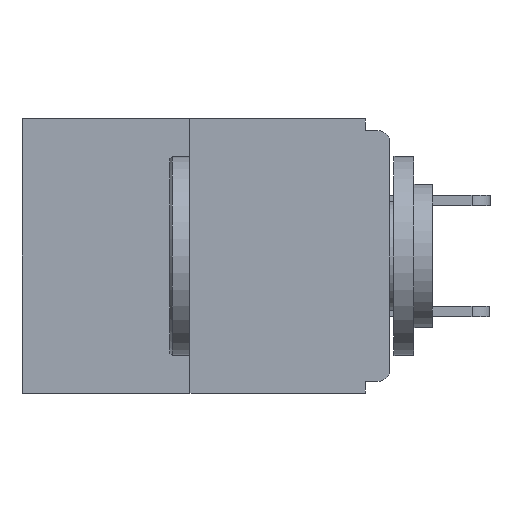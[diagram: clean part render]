
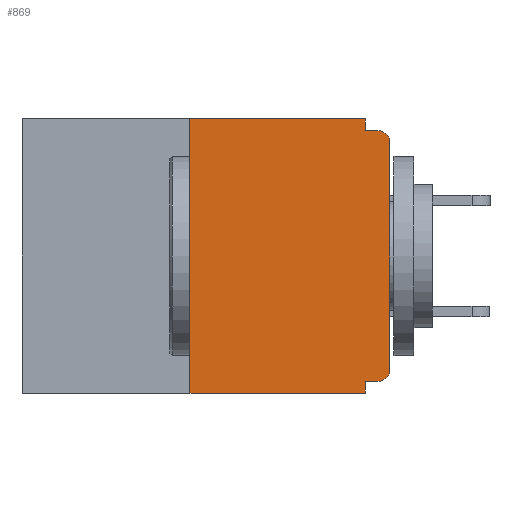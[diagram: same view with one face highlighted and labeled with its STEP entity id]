
A CAD part, left-side view. The second image highlights one B-rep face of the part: STEP entity #869.
In plain terms, the highlighted planar face has unit normal (-1, 0, 0).
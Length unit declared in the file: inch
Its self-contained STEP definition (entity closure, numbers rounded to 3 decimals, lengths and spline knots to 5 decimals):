
#82 = DIRECTION ( 'NONE',  ( 0., -1., 0. ) ) ;
#92 = ORIENTED_EDGE ( 'NONE', *, *, #14170, .T. ) ;
#514 = DIRECTION ( 'NONE',  ( 0., 0., -1. ) ) ;
#869 = ADVANCED_FACE ( 'NONE', ( #8161 ), #7181, .F. ) ;
#1082 = VECTOR ( 'NONE', #12350, 39.37008 ) ;
#1517 = VECTOR ( 'NONE', #14670, 39.37008 ) ;
#1728 = AXIS2_PLACEMENT_3D ( 'NONE', #14486, #8746, #17326 ) ;
#1764 = DIRECTION ( 'NONE',  ( -1., 0., 0. ) ) ;
#2073 = CARTESIAN_POINT ( 'NONE',  ( 0., 0.031, 0. ) ) ;
#2303 = LINE ( 'NONE', #11290, #13924 ) ;
#2343 = CARTESIAN_POINT ( 'NONE',  ( 0., 0.46, -0.343 ) ) ;
#2442 = EDGE_CURVE ( 'NONE', #13211, #17263, #9874, .T. ) ;
#2461 = AXIS2_PLACEMENT_3D ( 'NONE', #17201, #5905, #3043 ) ;
#2674 = VECTOR ( 'NONE', #3726, 39.37008 ) ;
#2774 = ORIENTED_EDGE ( 'NONE', *, *, #2442, .T. ) ;
#3043 = DIRECTION ( 'NONE',  ( 0., 0., -1. ) ) ;
#3223 = VECTOR ( 'NONE', #10202, 39.37008 ) ;
#3483 = CARTESIAN_POINT ( 'NONE',  ( 0., 0.031, -0.343 ) ) ;
#3511 = CARTESIAN_POINT ( 'NONE',  ( 0., 0.46, 0. ) ) ;
#3658 = CARTESIAN_POINT ( 'NONE',  ( 0., 0.25, 0. ) ) ;
#3726 = DIRECTION ( 'NONE',  ( 0., 0., 1. ) ) ;
#4218 = LINE ( 'NONE', #3658, #2674 ) ;
#4371 = CARTESIAN_POINT ( 'NONE',  ( 0., 0.25, -0.343 ) ) ;
#4703 = CARTESIAN_POINT ( 'NONE',  ( 0., 0., -0.328 ) ) ;
#4836 = EDGE_CURVE ( 'NONE', #18146, #11204, #14494, .T. ) ;
#5706 = CARTESIAN_POINT ( 'NONE',  ( 0., 0.031, -0.328 ) ) ;
#5816 = VERTEX_POINT ( 'NONE', #4371 ) ;
#5905 = DIRECTION ( 'NONE',  ( -1., 0., 0. ) ) ;
#5981 = CARTESIAN_POINT ( 'NONE',  ( 0., 0., -0.313 ) ) ;
#6450 = VECTOR ( 'NONE', #12423, 39.37008 ) ;
#7181 = PLANE ( 'NONE',  #1728 ) ;
#7378 = VECTOR ( 'NONE', #15451, 39.37008 ) ;
#7770 = DIRECTION ( 'NONE',  ( 0., -1., 0. ) ) ;
#7812 = LINE ( 'NONE', #4703, #1517 ) ;
#8161 = FACE_OUTER_BOUND ( 'NONE', #9070, .T. ) ;
#8279 = CARTESIAN_POINT ( 'NONE',  ( 0., 0.031, 0. ) ) ;
#8521 = EDGE_CURVE ( 'NONE', #18119, #12686, #9248, .T. ) ;
#8746 = DIRECTION ( 'NONE',  ( 1., 0., 0. ) ) ;
#8835 = CARTESIAN_POINT ( 'NONE',  ( 0., 0., 0. ) ) ;
#8848 = EDGE_CURVE ( 'NONE', #9846, #17263, #2303, .T. ) ;
#9070 = EDGE_LOOP ( 'NONE', ( #9831, #10696, #92, #11551, #13028, #14456, #15803, #2774, #17605, #9783 ) ) ;
#9082 = CARTESIAN_POINT ( 'NONE',  ( 0., 0.031, -0.015 ) ) ;
#9248 = LINE ( 'NONE', #3511, #14383 ) ;
#9339 = CARTESIAN_POINT ( 'NONE',  ( 0., 0.015, -0.328 ) ) ;
#9377 = LINE ( 'NONE', #2343, #1082 ) ;
#9783 = ORIENTED_EDGE ( 'NONE', *, *, #13656, .F. ) ;
#9831 = ORIENTED_EDGE ( 'NONE', *, *, #8521, .F. ) ;
#9846 = VERTEX_POINT ( 'NONE', #9082 ) ;
#9874 = CIRCLE ( 'NONE', #17698, 0.015 ) ;
#10202 = DIRECTION ( 'NONE',  ( 0., 0., 1. ) ) ;
#10339 = CARTESIAN_POINT ( 'NONE',  ( 0., 0.015, -0.03 ) ) ;
#10652 = EDGE_CURVE ( 'NONE', #11870, #18146, #7812, .T. ) ;
#10696 = ORIENTED_EDGE ( 'NONE', *, *, #13470, .F. ) ;
#10851 = CARTESIAN_POINT ( 'NONE',  ( 0., 0.031, -0.343 ) ) ;
#10976 = EDGE_CURVE ( 'NONE', #11870, #16475, #16549, .T. ) ;
#11204 = VERTEX_POINT ( 'NONE', #3483 ) ;
#11290 = CARTESIAN_POINT ( 'NONE',  ( 0., 0., -0.015 ) ) ;
#11551 = ORIENTED_EDGE ( 'NONE', *, *, #4836, .F. ) ;
#11870 = VERTEX_POINT ( 'NONE', #9339 ) ;
#12014 = CARTESIAN_POINT ( 'NONE',  ( 0., 0., -0.03 ) ) ;
#12350 = DIRECTION ( 'NONE',  ( 0., -1., 0. ) ) ;
#12423 = DIRECTION ( 'NONE',  ( 0., 0., -1. ) ) ;
#12686 = VERTEX_POINT ( 'NONE', #2073 ) ;
#13028 = ORIENTED_EDGE ( 'NONE', *, *, #10652, .F. ) ;
#13211 = VERTEX_POINT ( 'NONE', #12014 ) ;
#13292 = LINE ( 'NONE', #8835, #3223 ) ;
#13470 = EDGE_CURVE ( 'NONE', #5816, #18119, #4218, .T. ) ;
#13656 = EDGE_CURVE ( 'NONE', #12686, #9846, #15001, .T. ) ;
#13924 = VECTOR ( 'NONE', #82, 39.37008 ) ;
#14088 = CARTESIAN_POINT ( 'NONE',  ( 0., 0.25, 0. ) ) ;
#14170 = EDGE_CURVE ( 'NONE', #5816, #11204, #9377, .T. ) ;
#14383 = VECTOR ( 'NONE', #7770, 39.37008 ) ;
#14456 = ORIENTED_EDGE ( 'NONE', *, *, #10976, .T. ) ;
#14486 = CARTESIAN_POINT ( 'NONE',  ( 0., 0.46, 0. ) ) ;
#14494 = LINE ( 'NONE', #10851, #6450 ) ;
#14670 = DIRECTION ( 'NONE',  ( 0., 1., 0. ) ) ;
#15001 = LINE ( 'NONE', #8279, #7378 ) ;
#15451 = DIRECTION ( 'NONE',  ( 0., 0., -1. ) ) ;
#15803 = ORIENTED_EDGE ( 'NONE', *, *, #16251, .T. ) ;
#15976 = CARTESIAN_POINT ( 'NONE',  ( 0., 0.015, -0.015 ) ) ;
#16251 = EDGE_CURVE ( 'NONE', #16475, #13211, #13292, .T. ) ;
#16475 = VERTEX_POINT ( 'NONE', #5981 ) ;
#16549 = CIRCLE ( 'NONE', #2461, 0.015 ) ;
#17201 = CARTESIAN_POINT ( 'NONE',  ( 0., 0.015, -0.313 ) ) ;
#17263 = VERTEX_POINT ( 'NONE', #15976 ) ;
#17326 = DIRECTION ( 'NONE',  ( 0., 0., -1. ) ) ;
#17605 = ORIENTED_EDGE ( 'NONE', *, *, #8848, .F. ) ;
#17698 = AXIS2_PLACEMENT_3D ( 'NONE', #10339, #1764, #514 ) ;
#18119 = VERTEX_POINT ( 'NONE', #14088 ) ;
#18146 = VERTEX_POINT ( 'NONE', #5706 ) ;
